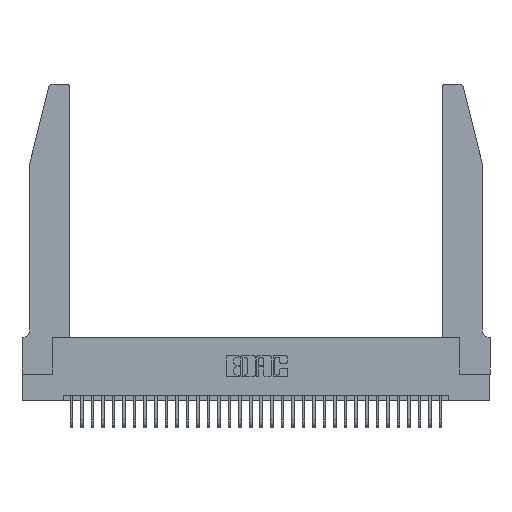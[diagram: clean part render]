
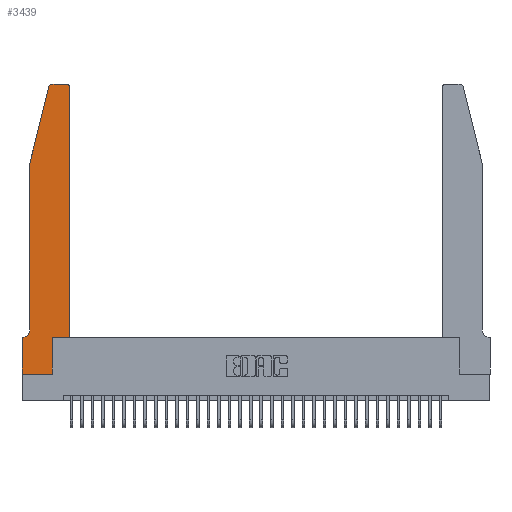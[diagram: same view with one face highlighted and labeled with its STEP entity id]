
A CAD part, top view. The second image highlights one B-rep face of the part: STEP entity #3439.
In plain terms, the highlighted planar face has unit normal (0, 0, 1).
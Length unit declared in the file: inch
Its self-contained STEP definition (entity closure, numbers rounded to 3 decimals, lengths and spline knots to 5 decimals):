
#670 = VECTOR ( 'NONE', #3035, 39.37008 ) ;
#1235 = CIRCLE ( 'NONE', #3020, 0.03 ) ;
#1367 = VERTEX_POINT ( 'NONE', #1831 ) ;
#1554 = LINE ( 'NONE', #32793, #15430 ) ;
#1575 = VERTEX_POINT ( 'NONE', #19706 ) ;
#1831 = CARTESIAN_POINT ( 'NONE',  ( 0., 0.35, 0.37 ) ) ;
#2368 = CARTESIAN_POINT ( 'NONE',  ( 0.0055, 0.35, 0.37 ) ) ;
#2963 = CARTESIAN_POINT ( 'NONE',  ( 0.4205, 2.75, 0.37 ) ) ;
#3020 = AXIS2_PLACEMENT_3D ( 'NONE', #21251, #4835, #24002 ) ;
#3035 = DIRECTION ( 'NONE',  ( 0., -1., 0. ) ) ;
#3354 = VERTEX_POINT ( 'NONE', #30277 ) ;
#3439 = ADVANCED_FACE ( 'NONE', ( #31195 ), #6268, .T. ) ;
#3616 = CARTESIAN_POINT ( 'NONE',  ( 0.0055, 0.42, 0.37 ) ) ;
#4052 = ORIENTED_EDGE ( 'NONE', *, *, #21554, .T. ) ;
#4117 = VERTEX_POINT ( 'NONE', #14541 ) ;
#4835 = DIRECTION ( 'NONE',  ( 0., 0., 1. ) ) ;
#4856 = EDGE_CURVE ( 'NONE', #24333, #1367, #24341, .T. ) ;
#6268 = PLANE ( 'NONE',  #29317 ) ;
#6387 = DIRECTION ( 'NONE',  ( -1., 0., 0. ) ) ;
#6663 = ORIENTED_EDGE ( 'NONE', *, *, #18598, .T. ) ;
#6849 = DIRECTION ( 'NONE',  ( 1., 0., 0. ) ) ;
#7029 = AXIS2_PLACEMENT_3D ( 'NONE', #11503, #30541, #14255 ) ;
#8071 = CARTESIAN_POINT ( 'NONE',  ( 0., 0., 0.37 ) ) ;
#8083 = LINE ( 'NONE', #22247, #670 ) ;
#8381 = ORIENTED_EDGE ( 'NONE', *, *, #23855, .T. ) ;
#8806 = ORIENTED_EDGE ( 'NONE', *, *, #14612, .T. ) ;
#10767 = VECTOR ( 'NONE', #25575, 39.37008 ) ;
#11503 = CARTESIAN_POINT ( 'NONE',  ( 0.4205, 2.72, 0.37 ) ) ;
#11667 = CARTESIAN_POINT ( 'NONE',  ( 0.0755, 2., 0.37 ) ) ;
#11848 = DIRECTION ( 'NONE',  ( 0., 0., 1. ) ) ;
#12127 = CARTESIAN_POINT ( 'NONE',  ( 0.0755, 0.35, 0.37 ) ) ;
#12185 = EDGE_CURVE ( 'NONE', #23462, #21793, #19318, .T. ) ;
#12739 = ORIENTED_EDGE ( 'NONE', *, *, #34199, .T. ) ;
#12982 = DIRECTION ( 'NONE',  ( 1., 0., 0. ) ) ;
#12987 = VECTOR ( 'NONE', #6849, 39.37008 ) ;
#13177 = CARTESIAN_POINT ( 'NONE',  ( 0.2865, 0., 0.37 ) ) ;
#14255 = DIRECTION ( 'NONE',  ( 1., 0., 0. ) ) ;
#14437 = ORIENTED_EDGE ( 'NONE', *, *, #12185, .T. ) ;
#14541 = CARTESIAN_POINT ( 'NONE',  ( 0.2865, 0.35, 0.37 ) ) ;
#14612 = EDGE_CURVE ( 'NONE', #21793, #3354, #18028, .T. ) ;
#14634 = CARTESIAN_POINT ( 'NONE',  ( 0.2605, 2.75, 0.37 ) ) ;
#14869 = VERTEX_POINT ( 'NONE', #13177 ) ;
#15039 = CARTESIAN_POINT ( 'NONE',  ( 0.4505, 0.35, 0.37 ) ) ;
#15430 = VECTOR ( 'NONE', #22891, 39.37008 ) ;
#16243 = VECTOR ( 'NONE', #20329, 39.37008 ) ;
#16891 = VERTEX_POINT ( 'NONE', #27668 ) ;
#17341 = CIRCLE ( 'NONE', #28219, 0.07 ) ;
#17401 = EDGE_LOOP ( 'NONE', ( #8806, #4052, #18679, #20380, #6663, #21224, #8381, #31028, #31900, #12739, #27191, #14437 ) ) ;
#18004 = CARTESIAN_POINT ( 'NONE',  ( 0.4505, 0.35, 0.37 ) ) ;
#18028 = LINE ( 'NONE', #14634, #10767 ) ;
#18130 = DIRECTION ( 'NONE',  ( 0., 1., 0. ) ) ;
#18328 = VECTOR ( 'NONE', #18130, 39.37008 ) ;
#18598 = EDGE_CURVE ( 'NONE', #30183, #24333, #17341, .T. ) ;
#18679 = ORIENTED_EDGE ( 'NONE', *, *, #29932, .T. ) ;
#19144 = LINE ( 'NONE', #18004, #18328 ) ;
#19318 = CIRCLE ( 'NONE', #7029, 0.03 ) ;
#19706 = CARTESIAN_POINT ( 'NONE',  ( 0.25487, 2.72718, 0.37 ) ) ;
#20329 = DIRECTION ( 'NONE',  ( -1., 0., 0. ) ) ;
#20380 = ORIENTED_EDGE ( 'NONE', *, *, #31451, .T. ) ;
#20946 = DIRECTION ( 'NONE',  ( -0.239, -0.971, 0. ) ) ;
#21224 = ORIENTED_EDGE ( 'NONE', *, *, #4856, .T. ) ;
#21251 = CARTESIAN_POINT ( 'NONE',  ( 0.284, 2.72, 0.37 ) ) ;
#21554 = EDGE_CURVE ( 'NONE', #3354, #1575, #1235, .T. ) ;
#21793 = VERTEX_POINT ( 'NONE', #2963 ) ;
#21972 = CARTESIAN_POINT ( 'NONE',  ( 0.2865, 0.35, 0.37 ) ) ;
#22216 = CARTESIAN_POINT ( 'NONE',  ( 0.0755, 0.42, 0.37 ) ) ;
#22247 = CARTESIAN_POINT ( 'NONE',  ( 0.0755, 2., 0.37 ) ) ;
#22472 = VERTEX_POINT ( 'NONE', #11667 ) ;
#22807 = DIRECTION ( 'NONE',  ( 0., 0., -1. ) ) ;
#22891 = DIRECTION ( 'NONE',  ( 0., -1., 0. ) ) ;
#23091 = CARTESIAN_POINT ( 'NONE',  ( 0.4505, 2.72, 0.37 ) ) ;
#23462 = VERTEX_POINT ( 'NONE', #23091 ) ;
#23855 = EDGE_CURVE ( 'NONE', #1367, #35423, #1554, .T. ) ;
#24002 = DIRECTION ( 'NONE',  ( 1., 0., 0. ) ) ;
#24333 = VERTEX_POINT ( 'NONE', #2368 ) ;
#24341 = LINE ( 'NONE', #12127, #16243 ) ;
#24714 = DIRECTION ( 'NONE',  ( 0., 1., 0. ) ) ;
#24858 = VECTOR ( 'NONE', #12982, 39.37008 ) ;
#25575 = DIRECTION ( 'NONE',  ( -1., 0., 0. ) ) ;
#25669 = EDGE_CURVE ( 'NONE', #14869, #4117, #29742, .T. ) ;
#25712 = LINE ( 'NONE', #29271, #24858 ) ;
#27191 = ORIENTED_EDGE ( 'NONE', *, *, #32534, .T. ) ;
#27362 = VECTOR ( 'NONE', #20946, 39.37008 ) ;
#27668 = CARTESIAN_POINT ( 'NONE',  ( 0.4505, 0.35, 0.37 ) ) ;
#28125 = CARTESIAN_POINT ( 'NONE',  ( 0., 0.35, 0.37 ) ) ;
#28219 = AXIS2_PLACEMENT_3D ( 'NONE', #3616, #22807, #6387 ) ;
#28302 = LINE ( 'NONE', #15039, #12987 ) ;
#28903 = VECTOR ( 'NONE', #24714, 39.37008 ) ;
#29271 = CARTESIAN_POINT ( 'NONE',  ( 0., 0., 0.37 ) ) ;
#29317 = AXIS2_PLACEMENT_3D ( 'NONE', #28125, #11848, #30883 ) ;
#29742 = LINE ( 'NONE', #21972, #28903 ) ;
#29932 = EDGE_CURVE ( 'NONE', #1575, #22472, #34620, .T. ) ;
#30183 = VERTEX_POINT ( 'NONE', #22216 ) ;
#30277 = CARTESIAN_POINT ( 'NONE',  ( 0.284, 2.75, 0.37 ) ) ;
#30541 = DIRECTION ( 'NONE',  ( 0., 0., 1. ) ) ;
#30883 = DIRECTION ( 'NONE',  ( 1., 0., 0. ) ) ;
#31028 = ORIENTED_EDGE ( 'NONE', *, *, #34751, .T. ) ;
#31195 = FACE_OUTER_BOUND ( 'NONE', #17401, .T. ) ;
#31451 = EDGE_CURVE ( 'NONE', #22472, #30183, #8083, .T. ) ;
#31900 = ORIENTED_EDGE ( 'NONE', *, *, #25669, .T. ) ;
#32534 = EDGE_CURVE ( 'NONE', #16891, #23462, #19144, .T. ) ;
#32793 = CARTESIAN_POINT ( 'NONE',  ( 0., 0., 0.37 ) ) ;
#34199 = EDGE_CURVE ( 'NONE', #4117, #16891, #28302, .T. ) ;
#34493 = CARTESIAN_POINT ( 'NONE',  ( 0.0755, 2., 0.37 ) ) ;
#34620 = LINE ( 'NONE', #34493, #27362 ) ;
#34751 = EDGE_CURVE ( 'NONE', #35423, #14869, #25712, .T. ) ;
#35423 = VERTEX_POINT ( 'NONE', #8071 ) ;
